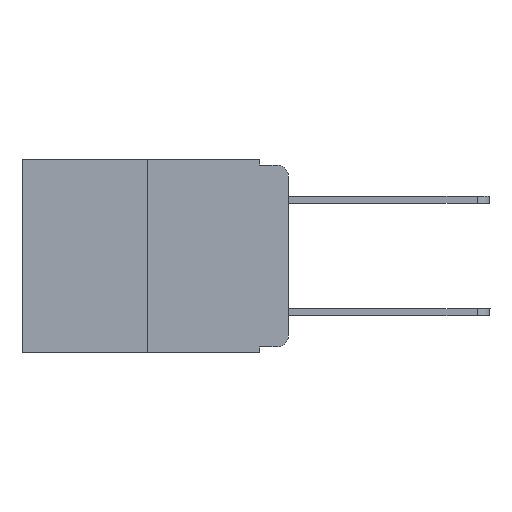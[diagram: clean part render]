
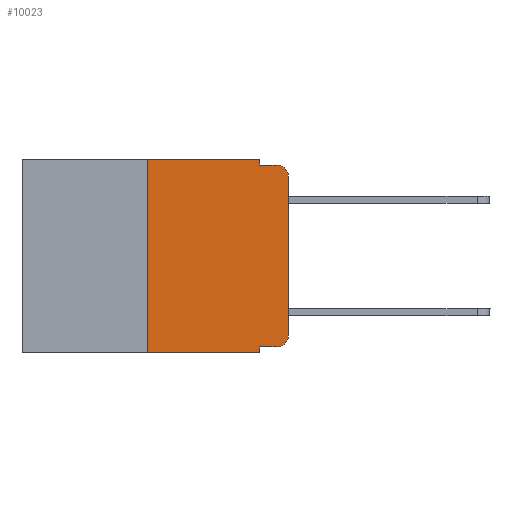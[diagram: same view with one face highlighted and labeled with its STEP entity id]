
A CAD part, left-side view. The second image highlights one B-rep face of the part: STEP entity #10023.
In plain terms, the highlighted planar face has unit normal (-1, 0, 0).
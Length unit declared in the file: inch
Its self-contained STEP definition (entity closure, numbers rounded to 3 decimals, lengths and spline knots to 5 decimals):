
#281 = VERTEX_POINT ( 'NONE', #6609 ) ;
#481 = CARTESIAN_POINT ( 'NONE',  ( 0., 0.473, 0. ) ) ;
#543 = ORIENTED_EDGE ( 'NONE', *, *, #10931, .T. ) ;
#737 = EDGE_CURVE ( 'NONE', #1242, #4290, #7493, .T. ) ;
#1242 = VERTEX_POINT ( 'NONE', #4830 ) ;
#1553 = VERTEX_POINT ( 'NONE', #4352 ) ;
#1575 = ORIENTED_EDGE ( 'NONE', *, *, #9933, .T. ) ;
#1757 = CARTESIAN_POINT ( 'NONE',  ( 0., 0.02, -0.333 ) ) ;
#1766 = ORIENTED_EDGE ( 'NONE', *, *, #8546, .T. ) ;
#1843 = VERTEX_POINT ( 'NONE', #7071 ) ;
#1861 = VECTOR ( 'NONE', #9083, 39.37008 ) ;
#1950 = DIRECTION ( 'NONE',  ( 0., -1., 0. ) ) ;
#2001 = EDGE_CURVE ( 'NONE', #1242, #1843, #6235, .T. ) ;
#2043 = ORIENTED_EDGE ( 'NONE', *, *, #7293, .F. ) ;
#2165 = DIRECTION ( 'NONE',  ( -1., 0., 0. ) ) ;
#2244 = VECTOR ( 'NONE', #1950, 39.37008 ) ;
#2627 = LINE ( 'NONE', #4140, #7945 ) ;
#2672 = LINE ( 'NONE', #5173, #5686 ) ;
#2684 = VERTEX_POINT ( 'NONE', #6412 ) ;
#2703 = EDGE_CURVE ( 'NONE', #1553, #281, #10016, .T. ) ;
#2828 = ORIENTED_EDGE ( 'NONE', *, *, #9776, .F. ) ;
#2929 = DIRECTION ( 'NONE',  ( 0., 0., -1. ) ) ;
#2940 = CARTESIAN_POINT ( 'NONE',  ( 0., 0.02, -0.03 ) ) ;
#2983 = CARTESIAN_POINT ( 'NONE',  ( 0., 0.25, -0.343 ) ) ;
#3089 = DIRECTION ( 'NONE',  ( 0., -1., 0. ) ) ;
#3232 = ORIENTED_EDGE ( 'NONE', *, *, #2001, .F. ) ;
#3275 = LINE ( 'NONE', #10159, #10389 ) ;
#3335 = DIRECTION ( 'NONE',  ( -1., 0., 0. ) ) ;
#3453 = VERTEX_POINT ( 'NONE', #9085 ) ;
#3762 = LINE ( 'NONE', #9111, #1861 ) ;
#3875 = CARTESIAN_POINT ( 'NONE',  ( 0., 0.051, 0. ) ) ;
#4047 = ORIENTED_EDGE ( 'NONE', *, *, #737, .T. ) ;
#4140 = CARTESIAN_POINT ( 'NONE',  ( 0., 0.473, 0. ) ) ;
#4290 = VERTEX_POINT ( 'NONE', #1757 ) ;
#4343 = CIRCLE ( 'NONE', #9183, 0.02 ) ;
#4352 = CARTESIAN_POINT ( 'NONE',  ( 0., 0.051, -0.01 ) ) ;
#4454 = VECTOR ( 'NONE', #7196, 39.37008 ) ;
#4579 = DIRECTION ( 'NONE',  ( 0., 0., -1. ) ) ;
#4830 = CARTESIAN_POINT ( 'NONE',  ( 0., 0.051, -0.333 ) ) ;
#5173 = CARTESIAN_POINT ( 'NONE',  ( 0., 0., 0. ) ) ;
#5667 = PLANE ( 'NONE',  #9647 ) ;
#5676 = VECTOR ( 'NONE', #2929, 39.37008 ) ;
#5686 = VECTOR ( 'NONE', #10408, 39.37008 ) ;
#5689 = ORIENTED_EDGE ( 'NONE', *, *, #2703, .F. ) ;
#6235 = LINE ( 'NONE', #3875, #5676 ) ;
#6311 = CARTESIAN_POINT ( 'NONE',  ( 0., 0.051, -0.01 ) ) ;
#6412 = CARTESIAN_POINT ( 'NONE',  ( 0., 0.25, 0. ) ) ;
#6456 = CARTESIAN_POINT ( 'NONE',  ( 0., 0.051, -0.333 ) ) ;
#6537 = DIRECTION ( 'NONE',  ( 0., 0., -1. ) ) ;
#6609 = CARTESIAN_POINT ( 'NONE',  ( 0., 0.02, -0.01 ) ) ;
#6780 = DIRECTION ( 'NONE',  ( 0., 0., -1. ) ) ;
#6918 = FACE_OUTER_BOUND ( 'NONE', #10201, .T. ) ;
#7005 = CARTESIAN_POINT ( 'NONE',  ( 0., 0., -0.313 ) ) ;
#7071 = CARTESIAN_POINT ( 'NONE',  ( 0., 0.051, -0.343 ) ) ;
#7193 = VERTEX_POINT ( 'NONE', #7005 ) ;
#7196 = DIRECTION ( 'NONE',  ( 0., 0., -1. ) ) ;
#7293 = EDGE_CURVE ( 'NONE', #2684, #8781, #2627, .T. ) ;
#7403 = DIRECTION ( 'NONE',  ( 1., 0., 0. ) ) ;
#7493 = LINE ( 'NONE', #6456, #10373 ) ;
#7559 = DIRECTION ( 'NONE',  ( 0., 0., 1. ) ) ;
#7648 = CARTESIAN_POINT ( 'NONE',  ( 0., 0.02, -0.313 ) ) ;
#7945 = VECTOR ( 'NONE', #8544, 39.37008 ) ;
#8007 = CIRCLE ( 'NONE', #9802, 0.02 ) ;
#8188 = EDGE_CURVE ( 'NONE', #8611, #2684, #3275, .T. ) ;
#8544 = DIRECTION ( 'NONE',  ( 0., -1., 0. ) ) ;
#8546 = EDGE_CURVE ( 'NONE', #3453, #281, #4343, .T. ) ;
#8611 = VERTEX_POINT ( 'NONE', #2983 ) ;
#8781 = VERTEX_POINT ( 'NONE', #9358 ) ;
#8823 = LINE ( 'NONE', #8905, #4454 ) ;
#8885 = ORIENTED_EDGE ( 'NONE', *, *, #10979, .T. ) ;
#8905 = CARTESIAN_POINT ( 'NONE',  ( 0., 0.051, 0. ) ) ;
#9083 = DIRECTION ( 'NONE',  ( 0., -1., 0. ) ) ;
#9085 = CARTESIAN_POINT ( 'NONE',  ( 0., 0., -0.03 ) ) ;
#9111 = CARTESIAN_POINT ( 'NONE',  ( 0., 0.473, -0.343 ) ) ;
#9183 = AXIS2_PLACEMENT_3D ( 'NONE', #2940, #2165, #4579 ) ;
#9358 = CARTESIAN_POINT ( 'NONE',  ( 0., 0.051, 0. ) ) ;
#9647 = AXIS2_PLACEMENT_3D ( 'NONE', #481, #7403, #6537 ) ;
#9776 = EDGE_CURVE ( 'NONE', #8781, #1553, #8823, .T. ) ;
#9802 = AXIS2_PLACEMENT_3D ( 'NONE', #7648, #3335, #6780 ) ;
#9933 = EDGE_CURVE ( 'NONE', #8611, #1843, #3762, .T. ) ;
#10016 = LINE ( 'NONE', #6311, #2244 ) ;
#10023 = ADVANCED_FACE ( 'NONE', ( #6918 ), #5667, .F. ) ;
#10159 = CARTESIAN_POINT ( 'NONE',  ( 0., 0.25, 0. ) ) ;
#10201 = EDGE_LOOP ( 'NONE', ( #8885, #1766, #5689, #2828, #2043, #10648, #1575, #3232, #4047, #543 ) ) ;
#10373 = VECTOR ( 'NONE', #3089, 39.37008 ) ;
#10389 = VECTOR ( 'NONE', #7559, 39.37008 ) ;
#10408 = DIRECTION ( 'NONE',  ( 0., 0., 1. ) ) ;
#10648 = ORIENTED_EDGE ( 'NONE', *, *, #8188, .F. ) ;
#10931 = EDGE_CURVE ( 'NONE', #4290, #7193, #8007, .T. ) ;
#10979 = EDGE_CURVE ( 'NONE', #7193, #3453, #2672, .T. ) ;
